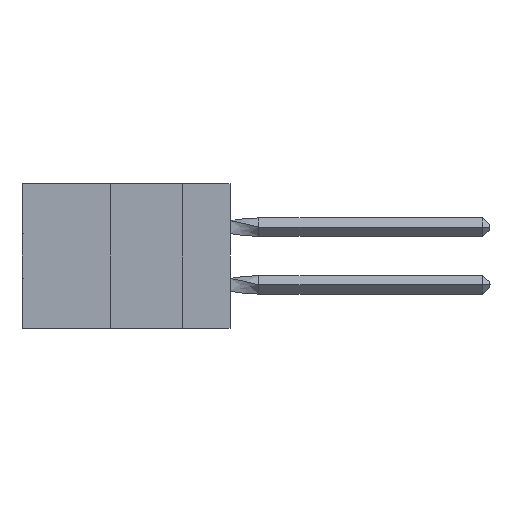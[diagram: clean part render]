
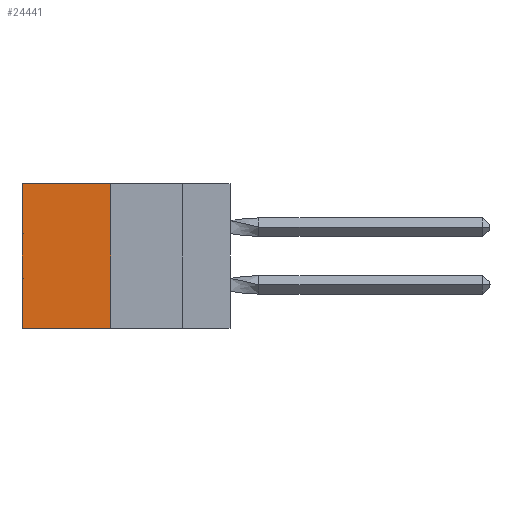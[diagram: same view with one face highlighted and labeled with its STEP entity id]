
A CAD part, left-side view. The second image highlights one B-rep face of the part: STEP entity #24441.
In plain terms, the highlighted planar face has unit normal (-1, 0, 0).
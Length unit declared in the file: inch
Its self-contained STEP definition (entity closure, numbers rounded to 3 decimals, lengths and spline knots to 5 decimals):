
#677 = LINE ( 'NONE', #2542, #34121 ) ;
#808 = LINE ( 'NONE', #8737, #24764 ) ;
#1370 = CARTESIAN_POINT ( 'NONE',  ( 0.305, 0.413, -0.5 ) ) ;
#1812 = VERTEX_POINT ( 'NONE', #1370 ) ;
#2542 = CARTESIAN_POINT ( 'NONE',  ( 0.305, 0.413, 0. ) ) ;
#2748 = CARTESIAN_POINT ( 'NONE',  ( 0.305, 0.413, 0. ) ) ;
#4119 = ORIENTED_EDGE ( 'NONE', *, *, #32519, .T. ) ;
#6891 = VECTOR ( 'NONE', #38742, 39.37008 ) ;
#8737 = CARTESIAN_POINT ( 'NONE',  ( 0.305, 0.413, -0.5 ) ) ;
#14067 = CARTESIAN_POINT ( 'NONE',  ( 0.305, 0.72, -0.5 ) ) ;
#14670 = VECTOR ( 'NONE', #24748, 39.37008 ) ;
#19094 = VERTEX_POINT ( 'NONE', #29856 ) ;
#21373 = LINE ( 'NONE', #45499, #6891 ) ;
#24441 = ADVANCED_FACE ( 'NONE', ( #35497 ), #27210, .F. ) ;
#24748 = DIRECTION ( 'NONE',  ( 0., 0., -1. ) ) ;
#24764 = VECTOR ( 'NONE', #33616, 39.37008 ) ;
#27063 = CARTESIAN_POINT ( 'NONE',  ( 0.305, 0.413, -0.5 ) ) ;
#27210 = PLANE ( 'NONE',  #31544 ) ;
#28046 = EDGE_CURVE ( 'NONE', #32275, #1812, #21373, .T. ) ;
#29856 = CARTESIAN_POINT ( 'NONE',  ( 0.305, 0.72, 0. ) ) ;
#30484 = DIRECTION ( 'NONE',  ( 0., 0., -1. ) ) ;
#31544 = AXIS2_PLACEMENT_3D ( 'NONE', #27063, #37685, #30484 ) ;
#32275 = VERTEX_POINT ( 'NONE', #2748 ) ;
#32462 = LINE ( 'NONE', #14067, #14670 ) ;
#32519 = EDGE_CURVE ( 'NONE', #19094, #40368, #32462, .T. ) ;
#32868 = EDGE_LOOP ( 'NONE', ( #4119, #41997, #38658, #37921 ) ) ;
#33429 = CARTESIAN_POINT ( 'NONE',  ( 0.305, 0.72, -0.5 ) ) ;
#33616 = DIRECTION ( 'NONE',  ( 0., 1., 0. ) ) ;
#34121 = VECTOR ( 'NONE', #34446, 39.37008 ) ;
#34446 = DIRECTION ( 'NONE',  ( 0., 1., 0. ) ) ;
#35497 = FACE_OUTER_BOUND ( 'NONE', #32868, .T. ) ;
#37685 = DIRECTION ( 'NONE',  ( 1., 0., 0. ) ) ;
#37921 = ORIENTED_EDGE ( 'NONE', *, *, #42875, .T. ) ;
#38658 = ORIENTED_EDGE ( 'NONE', *, *, #28046, .F. ) ;
#38742 = DIRECTION ( 'NONE',  ( 0., 0., -1. ) ) ;
#40368 = VERTEX_POINT ( 'NONE', #33429 ) ;
#41997 = ORIENTED_EDGE ( 'NONE', *, *, #44261, .F. ) ;
#42875 = EDGE_CURVE ( 'NONE', #32275, #19094, #677, .T. ) ;
#44261 = EDGE_CURVE ( 'NONE', #1812, #40368, #808, .T. ) ;
#45499 = CARTESIAN_POINT ( 'NONE',  ( 0.305, 0.413, -0.5 ) ) ;
